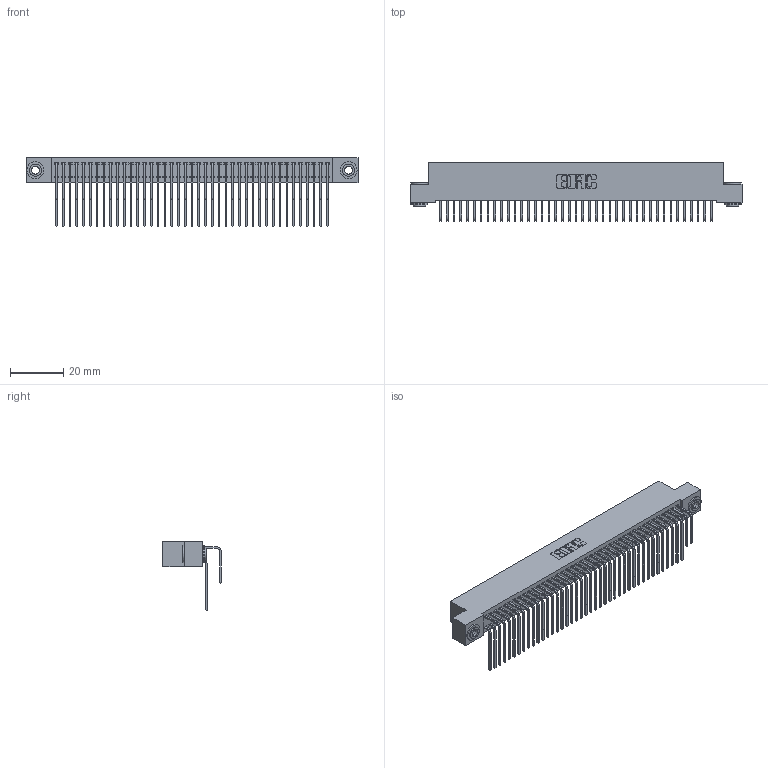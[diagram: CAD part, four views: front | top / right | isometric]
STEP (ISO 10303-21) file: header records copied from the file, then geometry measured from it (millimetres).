
FILE_DESCRIPTION (( 'STEP AP203' ), '1' );
FILE_NAME ('392-082-558-203.STEP', '2018-08-18T04:00:46', ( '' ), ( '' ), 'SwSTEP 2.0', 'SolidWorks 2016', '' );
FILE_SCHEMA (( 'CONFIG_CONTROL_DESIGN' ));
Length unit declared in the file: inch
Products named in the file (5): 392-082-558-203; 342 Part_.156 TH; 345-292-001_558 559 Tail - 1; 345-292-001_558 Tail - 2; 342-250-002_345-250-002-102
Assembly tree (85 placements, depth 2):
  392-082-558-203
    342 Part_.156 TH
    345-292-001_558 559 Tail - 1  x41
    345-292-001_558 Tail - 2  x41
    342-250-002_345-250-002-102  x2
Bounding box: 124.46 x 21.91 x 25.78 mm (x, y, z)
Volume: 11673.8 mm3; surface area: 21331.4 mm2
Topology: 85 solids, 85 shells, 4576 faces, 13577 edges, 8938 vertices
Faces by surface type: plane 3192, cylinder 1376, cone 8
Entity records: 28808 total; most frequent: CARTESIAN_POINT 4800, ORIENTED_EDGE 4678, DIRECTION 4117, EDGE_CURVE 2339, VECTOR 2147, LINE 2147, VERTEX_POINT 1554, AXIS2_PLACEMENT_3D 985
